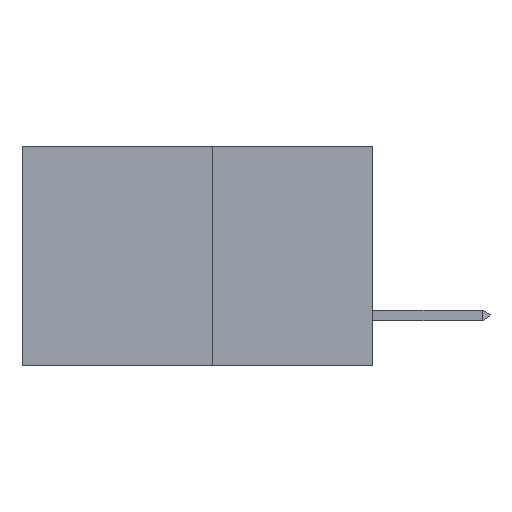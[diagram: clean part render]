
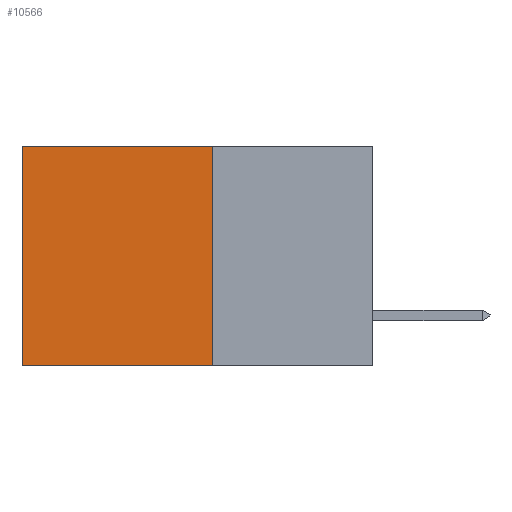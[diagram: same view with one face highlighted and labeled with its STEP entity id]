
A CAD part, left-side view. The second image highlights one B-rep face of the part: STEP entity #10566.
In plain terms, the highlighted planar face has unit normal (-1, 0, 0).
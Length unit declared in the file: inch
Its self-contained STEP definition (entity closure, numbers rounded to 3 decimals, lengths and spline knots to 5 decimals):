
#242 = EDGE_CURVE ( 'NONE', #9216, #2315, #13038, .T. ) ;
#285 = DIRECTION ( 'NONE',  ( 0., 1., 0. ) ) ;
#405 = CARTESIAN_POINT ( 'NONE',  ( 0.277, 0.27, -0.37 ) ) ;
#1643 = CARTESIAN_POINT ( 'NONE',  ( 0.277, 0.27, 0. ) ) ;
#1687 = DIRECTION ( 'NONE',  ( 0., 1., 0. ) ) ;
#1909 = ORIENTED_EDGE ( 'NONE', *, *, #11183, .T. ) ;
#2315 = VERTEX_POINT ( 'NONE', #10456 ) ;
#2950 = CARTESIAN_POINT ( 'NONE',  ( 0.277, 0.27, -0.37 ) ) ;
#3451 = ORIENTED_EDGE ( 'NONE', *, *, #242, .T. ) ;
#3638 = AXIS2_PLACEMENT_3D ( 'NONE', #2950, #4347, #13441 ) ;
#4347 = DIRECTION ( 'NONE',  ( 1., 0., 0. ) ) ;
#4553 = CARTESIAN_POINT ( 'NONE',  ( 0.277, 0.27, -0.37 ) ) ;
#4554 = ORIENTED_EDGE ( 'NONE', *, *, #13271, .F. ) ;
#5133 = VECTOR ( 'NONE', #285, 39.37008 ) ;
#6214 = VECTOR ( 'NONE', #1687, 39.37008 ) ;
#6943 = VERTEX_POINT ( 'NONE', #13484 ) ;
#7019 = ORIENTED_EDGE ( 'NONE', *, *, #10055, .F. ) ;
#7046 = PLANE ( 'NONE',  #3638 ) ;
#8142 = EDGE_LOOP ( 'NONE', ( #1909, #7019, #4554, #3451 ) ) ;
#9027 = VERTEX_POINT ( 'NONE', #15668 ) ;
#9216 = VERTEX_POINT ( 'NONE', #9739 ) ;
#9550 = DIRECTION ( 'NONE',  ( 0., 0., -1. ) ) ;
#9633 = LINE ( 'NONE', #405, #15922 ) ;
#9711 = FACE_OUTER_BOUND ( 'NONE', #8142, .T. ) ;
#9739 = CARTESIAN_POINT ( 'NONE',  ( 0.277, 0.27, 0. ) ) ;
#10055 = EDGE_CURVE ( 'NONE', #9027, #6943, #12033, .T. ) ;
#10456 = CARTESIAN_POINT ( 'NONE',  ( 0.277, 0.59, 0. ) ) ;
#10566 = ADVANCED_FACE ( 'NONE', ( #9711 ), #7046, .F. ) ;
#11183 = EDGE_CURVE ( 'NONE', #2315, #6943, #13015, .T. ) ;
#12033 = LINE ( 'NONE', #4553, #5133 ) ;
#13015 = LINE ( 'NONE', #13367, #15998 ) ;
#13038 = LINE ( 'NONE', #1643, #6214 ) ;
#13271 = EDGE_CURVE ( 'NONE', #9216, #9027, #9633, .T. ) ;
#13367 = CARTESIAN_POINT ( 'NONE',  ( 0.277, 0.59, -0.37 ) ) ;
#13441 = DIRECTION ( 'NONE',  ( 0., 0., -1. ) ) ;
#13484 = CARTESIAN_POINT ( 'NONE',  ( 0.277, 0.59, -0.37 ) ) ;
#15668 = CARTESIAN_POINT ( 'NONE',  ( 0.277, 0.27, -0.37 ) ) ;
#15922 = VECTOR ( 'NONE', #16236, 39.37008 ) ;
#15998 = VECTOR ( 'NONE', #9550, 39.37008 ) ;
#16236 = DIRECTION ( 'NONE',  ( 0., 0., -1. ) ) ;
